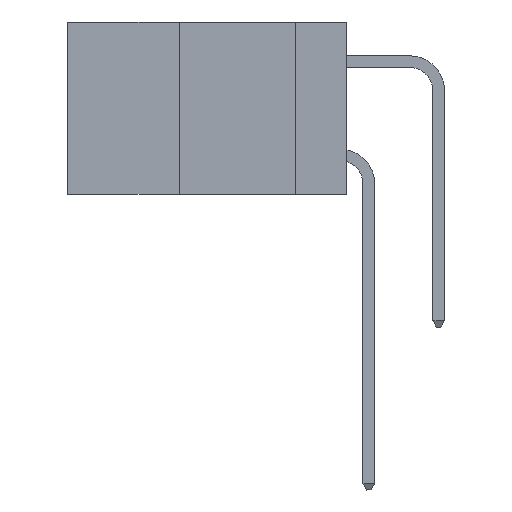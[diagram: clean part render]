
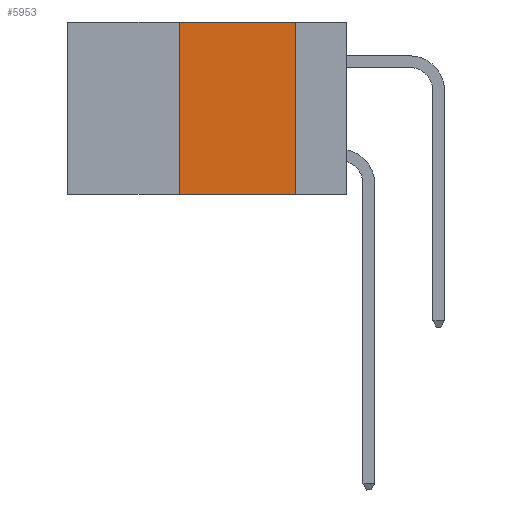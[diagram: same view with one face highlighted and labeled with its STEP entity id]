
A CAD part, left-side view. The second image highlights one B-rep face of the part: STEP entity #5953.
In plain terms, the highlighted planar face has unit normal (-1, 0, 0).
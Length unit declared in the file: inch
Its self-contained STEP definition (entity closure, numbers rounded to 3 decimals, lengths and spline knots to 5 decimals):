
#611 = LINE ( 'NONE', #5324, #654 ) ;
#654 = VECTOR ( 'NONE', #5251, 39.37008 ) ;
#728 = VECTOR ( 'NONE', #4607, 39.37008 ) ;
#796 = DIRECTION ( 'NONE',  ( 0., 0., 1. ) ) ;
#894 = VECTOR ( 'NONE', #3411, 39.37008 ) ;
#1065 = DIRECTION ( 'NONE',  ( 0., 0., -1. ) ) ;
#2016 = ORIENTED_EDGE ( 'NONE', *, *, #9427, .F. ) ;
#2308 = CARTESIAN_POINT ( 'NONE',  ( 0., 0.11, -0.37 ) ) ;
#3323 = LINE ( 'NONE', #10527, #728 ) ;
#3411 = DIRECTION ( 'NONE',  ( 0., 0., -1. ) ) ;
#3572 = EDGE_LOOP ( 'NONE', ( #2016, #5077, #9201, #4202 ) ) ;
#3936 = CARTESIAN_POINT ( 'NONE',  ( 0., 0.36, -0.37 ) ) ;
#4202 = ORIENTED_EDGE ( 'NONE', *, *, #9259, .T. ) ;
#4600 = CARTESIAN_POINT ( 'NONE',  ( 0., 0.36, 0. ) ) ;
#4607 = DIRECTION ( 'NONE',  ( 0., -1., 0. ) ) ;
#5077 = ORIENTED_EDGE ( 'NONE', *, *, #14331, .F. ) ;
#5251 = DIRECTION ( 'NONE',  ( 0., -1., 0. ) ) ;
#5324 = CARTESIAN_POINT ( 'NONE',  ( 0., 0.6, -0.37 ) ) ;
#5403 = CARTESIAN_POINT ( 'NONE',  ( 0., 0.11, 0. ) ) ;
#5713 = CARTESIAN_POINT ( 'NONE',  ( 0., 0.6, 0. ) ) ;
#5953 = ADVANCED_FACE ( 'NONE', ( #10125 ), #10343, .F. ) ;
#6026 = VERTEX_POINT ( 'NONE', #7812 ) ;
#6279 = VECTOR ( 'NONE', #796, 39.37008 ) ;
#6636 = LINE ( 'NONE', #4600, #6279 ) ;
#7812 = CARTESIAN_POINT ( 'NONE',  ( 0., 0.36, 0. ) ) ;
#9150 = LINE ( 'NONE', #5403, #894 ) ;
#9201 = ORIENTED_EDGE ( 'NONE', *, *, #11255, .F. ) ;
#9259 = EDGE_CURVE ( 'NONE', #11134, #11481, #611, .T. ) ;
#9427 = EDGE_CURVE ( 'NONE', #14073, #11481, #9150, .T. ) ;
#10125 = FACE_OUTER_BOUND ( 'NONE', #3572, .T. ) ;
#10343 = PLANE ( 'NONE',  #11668 ) ;
#10527 = CARTESIAN_POINT ( 'NONE',  ( 0., 0.6, 0. ) ) ;
#11134 = VERTEX_POINT ( 'NONE', #3936 ) ;
#11255 = EDGE_CURVE ( 'NONE', #11134, #6026, #6636, .T. ) ;
#11481 = VERTEX_POINT ( 'NONE', #2308 ) ;
#11668 = AXIS2_PLACEMENT_3D ( 'NONE', #5713, #15001, #1065 ) ;
#13226 = CARTESIAN_POINT ( 'NONE',  ( 0., 0.11, 0. ) ) ;
#14073 = VERTEX_POINT ( 'NONE', #13226 ) ;
#14331 = EDGE_CURVE ( 'NONE', #6026, #14073, #3323, .T. ) ;
#15001 = DIRECTION ( 'NONE',  ( 1., 0., 0. ) ) ;
